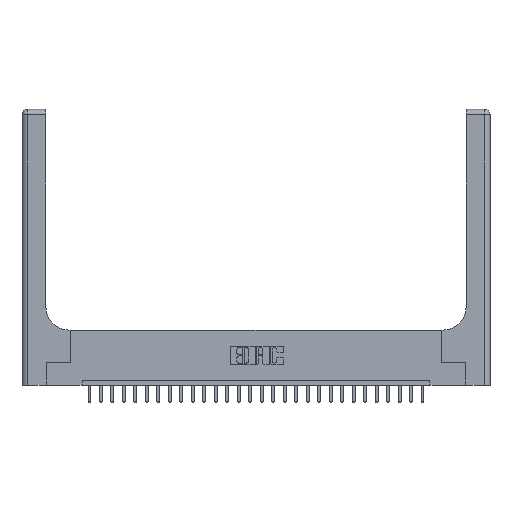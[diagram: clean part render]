
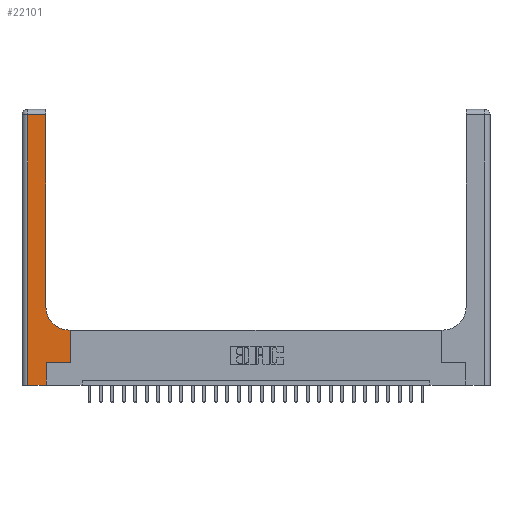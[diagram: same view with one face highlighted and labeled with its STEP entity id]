
A CAD part, top view. The second image highlights one B-rep face of the part: STEP entity #22101.
In plain terms, the highlighted planar face has unit normal (0, 0, 1).
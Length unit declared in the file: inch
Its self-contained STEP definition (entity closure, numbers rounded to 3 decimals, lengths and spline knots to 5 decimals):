
#135 = CARTESIAN_POINT ( 'NONE',  ( 0., 2.94, 0.37 ) ) ;
#323 = CARTESIAN_POINT ( 'NONE',  ( 0.265, 0.25, 0.37 ) ) ;
#368 = ORIENTED_EDGE ( 'NONE', *, *, #9162, .T. ) ;
#533 = DIRECTION ( 'NONE',  ( 0., 1., 0. ) ) ;
#1248 = CARTESIAN_POINT ( 'NONE',  ( 0.528, 0.6, 0.37 ) ) ;
#1485 = VERTEX_POINT ( 'NONE', #8625 ) ;
#1490 = CARTESIAN_POINT ( 'NONE',  ( 0.26, 2.94, 0.37 ) ) ;
#1524 = PLANE ( 'NONE',  #8243 ) ;
#2136 = CARTESIAN_POINT ( 'NONE',  ( 0.265, 0., 0.37 ) ) ;
#2451 = VERTEX_POINT ( 'NONE', #19407 ) ;
#2492 = LINE ( 'NONE', #18523, #14268 ) ;
#3456 = LINE ( 'NONE', #11716, #18853 ) ;
#4068 = CARTESIAN_POINT ( 'NONE',  ( 0.06, 0., 0.37 ) ) ;
#4723 = EDGE_CURVE ( 'NONE', #10912, #14513, #15520, .T. ) ;
#5528 = VECTOR ( 'NONE', #23292, 39.37008 ) ;
#5606 = LINE ( 'NONE', #6005, #8886 ) ;
#6005 = CARTESIAN_POINT ( 'NONE',  ( 0., 0., 0.37 ) ) ;
#7103 = ORIENTED_EDGE ( 'NONE', *, *, #19789, .T. ) ;
#7117 = VECTOR ( 'NONE', #16328, 39.37008 ) ;
#7575 = CARTESIAN_POINT ( 'NONE',  ( 0.265, 0., 0.37 ) ) ;
#7974 = DIRECTION ( 'NONE',  ( 0., -1., 0. ) ) ;
#8243 = AXIS2_PLACEMENT_3D ( 'NONE', #17291, #23742, #9153 ) ;
#8323 = LINE ( 'NONE', #2136, #7117 ) ;
#8333 = CIRCLE ( 'NONE', #11247, 0.25 ) ;
#8625 = CARTESIAN_POINT ( 'NONE',  ( 0.51, 0.6, 0.37 ) ) ;
#8886 = VECTOR ( 'NONE', #21499, 39.37008 ) ;
#9153 = DIRECTION ( 'NONE',  ( -1., 0., 0. ) ) ;
#9157 = LINE ( 'NONE', #13230, #18203 ) ;
#9162 = EDGE_CURVE ( 'NONE', #15927, #13272, #5606, .T. ) ;
#9485 = DIRECTION ( 'NONE',  ( 1., 0., 0. ) ) ;
#10174 = CARTESIAN_POINT ( 'NONE',  ( 0.06, 2.94, 0.37 ) ) ;
#10481 = ORIENTED_EDGE ( 'NONE', *, *, #17751, .T. ) ;
#10775 = ORIENTED_EDGE ( 'NONE', *, *, #11787, .T. ) ;
#10905 = CARTESIAN_POINT ( 'NONE',  ( 0.528, 0.25, 0.37 ) ) ;
#10912 = VERTEX_POINT ( 'NONE', #323 ) ;
#11238 = FACE_OUTER_BOUND ( 'NONE', #17440, .T. ) ;
#11247 = AXIS2_PLACEMENT_3D ( 'NONE', #13173, #19347, #9485 ) ;
#11716 = CARTESIAN_POINT ( 'NONE',  ( 0.26, 0.6, 0.37 ) ) ;
#11787 = EDGE_CURVE ( 'NONE', #20845, #18789, #24435, .T. ) ;
#11871 = DIRECTION ( 'NONE',  ( 0., 1., 0. ) ) ;
#13173 = CARTESIAN_POINT ( 'NONE',  ( 0.51, 0.85, 0.37 ) ) ;
#13230 = CARTESIAN_POINT ( 'NONE',  ( 0.06, 3., 0.37 ) ) ;
#13272 = VERTEX_POINT ( 'NONE', #7575 ) ;
#13363 = EDGE_CURVE ( 'NONE', #18789, #15927, #9157, .T. ) ;
#13743 = EDGE_CURVE ( 'NONE', #14513, #17413, #23843, .T. ) ;
#14268 = VECTOR ( 'NONE', #533, 39.37008 ) ;
#14513 = VERTEX_POINT ( 'NONE', #10905 ) ;
#14997 = CARTESIAN_POINT ( 'NONE',  ( 0.265, 0.25, 0.37 ) ) ;
#15520 = LINE ( 'NONE', #14997, #5528 ) ;
#15927 = VERTEX_POINT ( 'NONE', #4068 ) ;
#16328 = DIRECTION ( 'NONE',  ( 0., 1., 0. ) ) ;
#16950 = VECTOR ( 'NONE', #11871, 39.37008 ) ;
#17291 = CARTESIAN_POINT ( 'NONE',  ( 0., 3., 0.37 ) ) ;
#17413 = VERTEX_POINT ( 'NONE', #1248 ) ;
#17440 = EDGE_LOOP ( 'NONE', ( #7103, #10775, #20562, #368, #17733, #23399, #20724, #23594, #10481 ) ) ;
#17733 = ORIENTED_EDGE ( 'NONE', *, *, #20972, .T. ) ;
#17751 = EDGE_CURVE ( 'NONE', #1485, #2451, #8333, .T. ) ;
#17983 = DIRECTION ( 'NONE',  ( -1., 0., 0. ) ) ;
#18203 = VECTOR ( 'NONE', #7974, 39.37008 ) ;
#18523 = CARTESIAN_POINT ( 'NONE',  ( 0.26, 3., 0.37 ) ) ;
#18789 = VERTEX_POINT ( 'NONE', #10174 ) ;
#18853 = VECTOR ( 'NONE', #25794, 39.37008 ) ;
#19347 = DIRECTION ( 'NONE',  ( 0., 0., -1. ) ) ;
#19407 = CARTESIAN_POINT ( 'NONE',  ( 0.26, 0.85, 0.37 ) ) ;
#19789 = EDGE_CURVE ( 'NONE', #2451, #20845, #2492, .T. ) ;
#19872 = VECTOR ( 'NONE', #17983, 39.37008 ) ;
#20299 = EDGE_CURVE ( 'NONE', #17413, #1485, #3456, .T. ) ;
#20562 = ORIENTED_EDGE ( 'NONE', *, *, #13363, .T. ) ;
#20724 = ORIENTED_EDGE ( 'NONE', *, *, #13743, .T. ) ;
#20845 = VERTEX_POINT ( 'NONE', #1490 ) ;
#20972 = EDGE_CURVE ( 'NONE', #13272, #10912, #8323, .T. ) ;
#21499 = DIRECTION ( 'NONE',  ( 1., 0., 0. ) ) ;
#21865 = CARTESIAN_POINT ( 'NONE',  ( 0.528, 0.25, 0.37 ) ) ;
#22101 = ADVANCED_FACE ( 'NONE', ( #11238 ), #1524, .F. ) ;
#23292 = DIRECTION ( 'NONE',  ( 1., 0., 0. ) ) ;
#23399 = ORIENTED_EDGE ( 'NONE', *, *, #4723, .T. ) ;
#23594 = ORIENTED_EDGE ( 'NONE', *, *, #20299, .T. ) ;
#23742 = DIRECTION ( 'NONE',  ( 0., 0., -1. ) ) ;
#23843 = LINE ( 'NONE', #21865, #16950 ) ;
#24435 = LINE ( 'NONE', #135, #19872 ) ;
#25794 = DIRECTION ( 'NONE',  ( -1., 0., 0. ) ) ;
